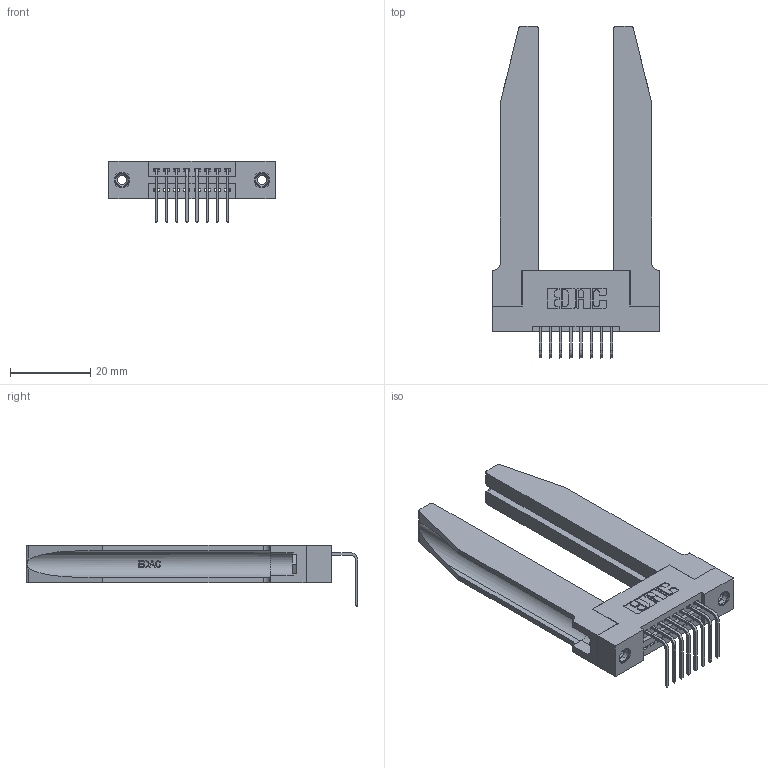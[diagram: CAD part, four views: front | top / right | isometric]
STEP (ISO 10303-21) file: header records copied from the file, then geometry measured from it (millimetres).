
FILE_DESCRIPTION (( 'STEP AP203' ), '1' );
FILE_NAME ('395-008-558-178.STEP', '2019-10-11T01:58:51', ( '' ), ( '' ), 'SwSTEP 2.0', 'SolidWorks 2016', '' );
FILE_SCHEMA (( 'CONFIG_CONTROL_DESIGN' ));
Length unit declared in the file: inch
Products named in the file (5): 345-292-001_558 Tail - 2; 345-250-001_345-250-001-102; 345-220-078_345-220-078; 395-008-558-178; 345 Part_Flush Mounting Lugs - 0.156 Dia-TH
Assembly tree (13 placements, depth 2):
  395-008-558-178
    345 Part_Flush Mounting Lugs - 0.156 Dia-TH
    345-292-001_558 Tail - 2  x8
    345-250-001_345-250-001-102  x2
    345-220-078_345-220-078  x2
Bounding box: 41.55 x 82.79 x 15.37 mm (x, y, z)
Volume: 11465.5 mm3; surface area: 11450.5 mm2
Topology: 13 solids, 13 shells, 840 faces, 2405 edges, 1582 vertices
Faces by surface type: plane 558, cylinder 230, bspline 36, cone 12, torus 4
Entity records: 15422 total; most frequent: CARTESIAN_POINT 3571, ORIENTED_EDGE 2410, DIRECTION 2175, EDGE_CURVE 1205, LINE 947, VECTOR 947, VERTEX_POINT 796, AXIS2_PLACEMENT_3D 614
